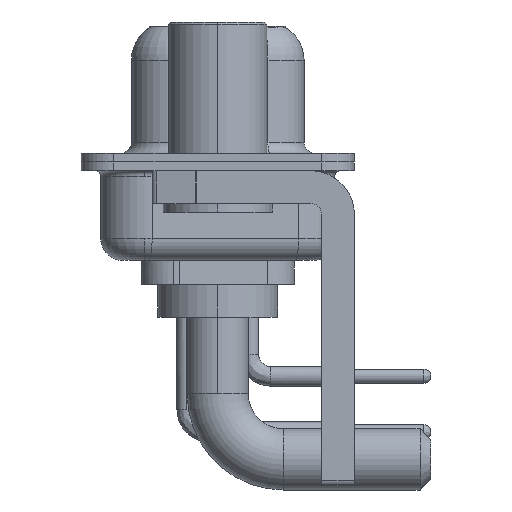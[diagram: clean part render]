
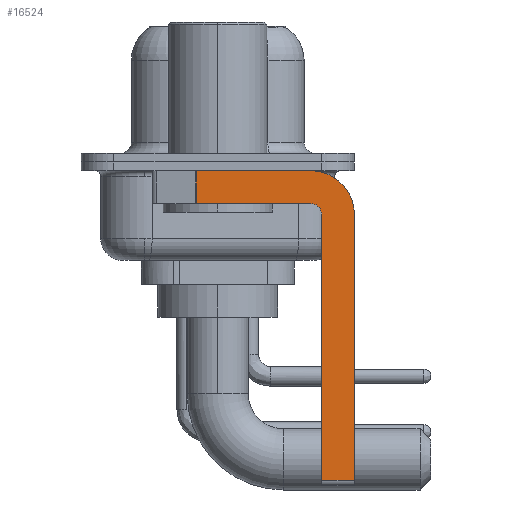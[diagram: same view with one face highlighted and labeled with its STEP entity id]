
A CAD part, left-side view. The second image highlights one B-rep face of the part: STEP entity #16524.
In plain terms, the highlighted planar face has unit normal (-1, 0, 0).
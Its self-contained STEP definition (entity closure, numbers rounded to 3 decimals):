
#174 = VECTOR ( 'NONE', #6242, 1000. ) ;
#241 = LINE ( 'NONE', #5017, #174 ) ;
#260 = ORIENTED_EDGE ( 'NONE', *, *, #1801, .F. ) ;
#695 = VERTEX_POINT ( 'NONE', #7577 ) ;
#1108 = AXIS2_PLACEMENT_3D ( 'NONE', #15742, #3402, #12716 ) ;
#1332 = DIRECTION ( 'NONE',  ( 0., -1., 0. ) ) ;
#1337 = DIRECTION ( 'NONE',  ( 1., 0., 0. ) ) ;
#1412 = ORIENTED_EDGE ( 'NONE', *, *, #9412, .T. ) ;
#1436 = CARTESIAN_POINT ( 'NONE',  ( -2.9, -4.75, -2.4 ) ) ;
#1801 = EDGE_CURVE ( 'NONE', #5484, #13662, #5629, .T. ) ;
#2482 = VERTEX_POINT ( 'NONE', #11044 ) ;
#2617 = ORIENTED_EDGE ( 'NONE', *, *, #5436, .T. ) ;
#3216 = VERTEX_POINT ( 'NONE', #13654 ) ;
#3402 = DIRECTION ( 'NONE',  ( -1., 0., 0. ) ) ;
#3917 = VERTEX_POINT ( 'NONE', #5275 ) ;
#3987 = VECTOR ( 'NONE', #11013, 1000. ) ;
#4339 = ORIENTED_EDGE ( 'NONE', *, *, #12341, .F. ) ;
#4461 = DIRECTION ( 'NONE',  ( 1., 0., 0. ) ) ;
#4566 = AXIS2_PLACEMENT_3D ( 'NONE', #7537, #1337, #5947 ) ;
#4734 = ORIENTED_EDGE ( 'NONE', *, *, #5448, .F. ) ;
#4879 = CARTESIAN_POINT ( 'NONE',  ( -2.9, -4.25, -1.9 ) ) ;
#5017 = CARTESIAN_POINT ( 'NONE',  ( -2.9, 0.978, -1.9 ) ) ;
#5275 = CARTESIAN_POINT ( 'NONE',  ( -2.9, 0.978, -1.9 ) ) ;
#5436 = EDGE_CURVE ( 'NONE', #5484, #3917, #241, .T. ) ;
#5448 = EDGE_CURVE ( 'NONE', #3216, #13180, #13759, .T. ) ;
#5484 = VERTEX_POINT ( 'NONE', #12822 ) ;
#5629 = LINE ( 'NONE', #19558, #18989 ) ;
#5947 = DIRECTION ( 'NONE',  ( 0., 0., -1. ) ) ;
#6084 = AXIS2_PLACEMENT_3D ( 'NONE', #15181, #4461, #14880 ) ;
#6232 = LINE ( 'NONE', #12327, #15189 ) ;
#6242 = DIRECTION ( 'NONE',  ( 0., 0., -1. ) ) ;
#6398 = EDGE_LOOP ( 'NONE', ( #260, #2617, #17402, #13527, #4734, #1412, #12406, #4339 ) ) ;
#7537 = CARTESIAN_POINT ( 'NONE',  ( -2.9, -4.25, -2.4 ) ) ;
#7577 = CARTESIAN_POINT ( 'NONE',  ( -2.9, -6.25, -2.4 ) ) ;
#7583 = CARTESIAN_POINT ( 'NONE',  ( -2.9, -6.25, -14.55 ) ) ;
#8756 = EDGE_CURVE ( 'NONE', #2482, #3917, #12290, .T. ) ;
#9412 = EDGE_CURVE ( 'NONE', #3216, #10535, #10226, .T. ) ;
#9708 = CIRCLE ( 'NONE', #1108, 0.5 ) ;
#10226 = LINE ( 'NONE', #16050, #19144 ) ;
#10535 = VERTEX_POINT ( 'NONE', #7583 ) ;
#11013 = DIRECTION ( 'NONE',  ( 0., 0., 1. ) ) ;
#11044 = CARTESIAN_POINT ( 'NONE',  ( -2.9, -4.25, -1.9 ) ) ;
#12234 = CARTESIAN_POINT ( 'NONE',  ( -2.9, -4.75, -14.8 ) ) ;
#12290 = LINE ( 'NONE', #4879, #17208 ) ;
#12327 = CARTESIAN_POINT ( 'NONE',  ( -2.9, -6.25, -2.4 ) ) ;
#12341 = EDGE_CURVE ( 'NONE', #13662, #695, #14703, .T. ) ;
#12406 = ORIENTED_EDGE ( 'NONE', *, *, #18087, .F. ) ;
#12716 = DIRECTION ( 'NONE',  ( 0., 0., 1. ) ) ;
#12822 = CARTESIAN_POINT ( 'NONE',  ( -2.9, 0.978, -0.4 ) ) ;
#13180 = VERTEX_POINT ( 'NONE', #1436 ) ;
#13527 = ORIENTED_EDGE ( 'NONE', *, *, #18009, .F. ) ;
#13554 = PLANE ( 'NONE',  #4566 ) ;
#13654 = CARTESIAN_POINT ( 'NONE',  ( -2.9, -4.75, -14.55 ) ) ;
#13662 = VERTEX_POINT ( 'NONE', #14834 ) ;
#13759 = LINE ( 'NONE', #12234, #3987 ) ;
#14703 = CIRCLE ( 'NONE', #6084, 2. ) ;
#14747 = DIRECTION ( 'NONE',  ( 0., -1., 0. ) ) ;
#14834 = CARTESIAN_POINT ( 'NONE',  ( -2.9, -4.25, -0.4 ) ) ;
#14880 = DIRECTION ( 'NONE',  ( 0., 0., -1. ) ) ;
#15181 = CARTESIAN_POINT ( 'NONE',  ( -2.9, -4.25, -2.4 ) ) ;
#15189 = VECTOR ( 'NONE', #18455, 1000. ) ;
#15742 = CARTESIAN_POINT ( 'NONE',  ( -2.9, -4.25, -2.4 ) ) ;
#16050 = CARTESIAN_POINT ( 'NONE',  ( -2.9, -4.25, -14.55 ) ) ;
#16524 = ADVANCED_FACE ( 'NONE', ( #19562 ), #13554, .F. ) ;
#17208 = VECTOR ( 'NONE', #18516, 1000. ) ;
#17402 = ORIENTED_EDGE ( 'NONE', *, *, #8756, .F. ) ;
#18009 = EDGE_CURVE ( 'NONE', #13180, #2482, #9708, .T. ) ;
#18087 = EDGE_CURVE ( 'NONE', #695, #10535, #6232, .T. ) ;
#18455 = DIRECTION ( 'NONE',  ( 0., 0., -1. ) ) ;
#18516 = DIRECTION ( 'NONE',  ( 0., 1., 0. ) ) ;
#18989 = VECTOR ( 'NONE', #1332, 1000. ) ;
#19144 = VECTOR ( 'NONE', #14747, 1000. ) ;
#19558 = CARTESIAN_POINT ( 'NONE',  ( -2.9, 3., -0.4 ) ) ;
#19562 = FACE_OUTER_BOUND ( 'NONE', #6398, .T. ) ;
